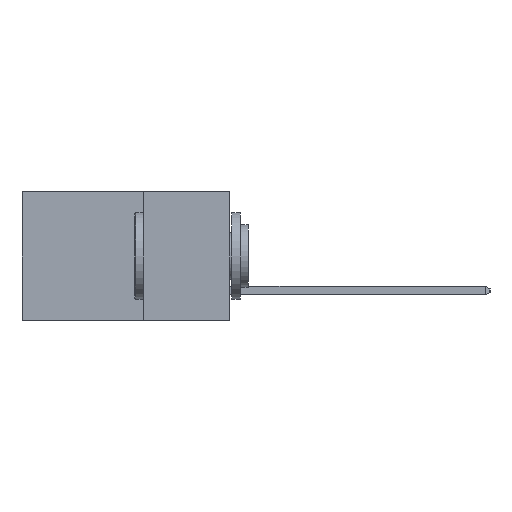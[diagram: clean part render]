
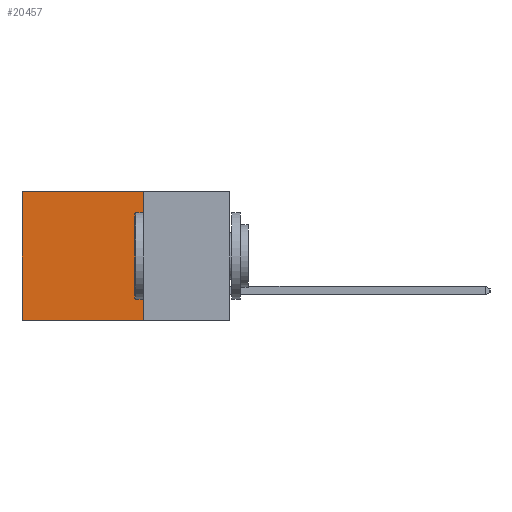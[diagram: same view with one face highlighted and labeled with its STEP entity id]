
A CAD part, left-side view. The second image highlights one B-rep face of the part: STEP entity #20457.
In plain terms, the highlighted planar face has unit normal (-1, 0, 0).
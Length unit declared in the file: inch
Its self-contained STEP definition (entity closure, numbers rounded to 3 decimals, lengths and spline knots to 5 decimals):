
#174 = VECTOR ( 'NONE', #1731, 39.37008 ) ;
#238 = LINE ( 'NONE', #1295, #17024 ) ;
#317 = FACE_OUTER_BOUND ( 'NONE', #6025, .T. ) ;
#446 = VECTOR ( 'NONE', #18456, 39.37008 ) ;
#925 = PLANE ( 'NONE',  #10501 ) ;
#1295 = CARTESIAN_POINT ( 'NONE',  ( 0.2615, 0.25, -0.37 ) ) ;
#1731 = DIRECTION ( 'NONE',  ( 0., 1., 0. ) ) ;
#4203 = DIRECTION ( 'NONE',  ( 0., 0., -1. ) ) ;
#4646 = VERTEX_POINT ( 'NONE', #11477 ) ;
#4741 = VERTEX_POINT ( 'NONE', #8588 ) ;
#4795 = LINE ( 'NONE', #18557, #446 ) ;
#5307 = EDGE_CURVE ( 'NONE', #14623, #4741, #4795, .T. ) ;
#6025 = EDGE_LOOP ( 'NONE', ( #20415, #18345, #9107, #18813 ) ) ;
#6515 = CARTESIAN_POINT ( 'NONE',  ( 0.2615, 0.6, 0. ) ) ;
#8588 = CARTESIAN_POINT ( 'NONE',  ( 0.2615, 0.6, -0.37 ) ) ;
#8979 = LINE ( 'NONE', #17924, #174 ) ;
#9107 = ORIENTED_EDGE ( 'NONE', *, *, #9794, .F. ) ;
#9794 = EDGE_CURVE ( 'NONE', #10165, #4646, #10974, .T. ) ;
#10165 = VERTEX_POINT ( 'NONE', #12063 ) ;
#10501 = AXIS2_PLACEMENT_3D ( 'NONE', #17129, #14017, #4203 ) ;
#10974 = LINE ( 'NONE', #15798, #18846 ) ;
#11477 = CARTESIAN_POINT ( 'NONE',  ( 0.2615, 0.25, -0.37 ) ) ;
#12063 = CARTESIAN_POINT ( 'NONE',  ( 0.2615, 0.25, 0. ) ) ;
#13753 = EDGE_CURVE ( 'NONE', #4646, #4741, #238, .T. ) ;
#14017 = DIRECTION ( 'NONE',  ( 1., 0., 0. ) ) ;
#14623 = VERTEX_POINT ( 'NONE', #6515 ) ;
#15708 = DIRECTION ( 'NONE',  ( 0., 0., -1. ) ) ;
#15798 = CARTESIAN_POINT ( 'NONE',  ( 0.2615, 0.25, -0.37 ) ) ;
#17024 = VECTOR ( 'NONE', #17558, 39.37008 ) ;
#17129 = CARTESIAN_POINT ( 'NONE',  ( 0.2615, 0.25, -0.37 ) ) ;
#17138 = EDGE_CURVE ( 'NONE', #10165, #14623, #8979, .T. ) ;
#17558 = DIRECTION ( 'NONE',  ( 0., 1., 0. ) ) ;
#17924 = CARTESIAN_POINT ( 'NONE',  ( 0.2615, 0.25, 0. ) ) ;
#18345 = ORIENTED_EDGE ( 'NONE', *, *, #13753, .F. ) ;
#18456 = DIRECTION ( 'NONE',  ( 0., 0., -1. ) ) ;
#18557 = CARTESIAN_POINT ( 'NONE',  ( 0.2615, 0.6, -0.37 ) ) ;
#18813 = ORIENTED_EDGE ( 'NONE', *, *, #17138, .T. ) ;
#18846 = VECTOR ( 'NONE', #15708, 39.37008 ) ;
#20415 = ORIENTED_EDGE ( 'NONE', *, *, #5307, .T. ) ;
#20457 = ADVANCED_FACE ( 'NONE', ( #317 ), #925, .F. ) ;
